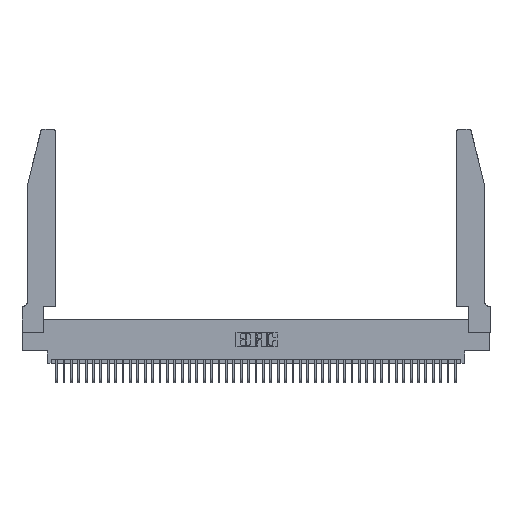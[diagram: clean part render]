
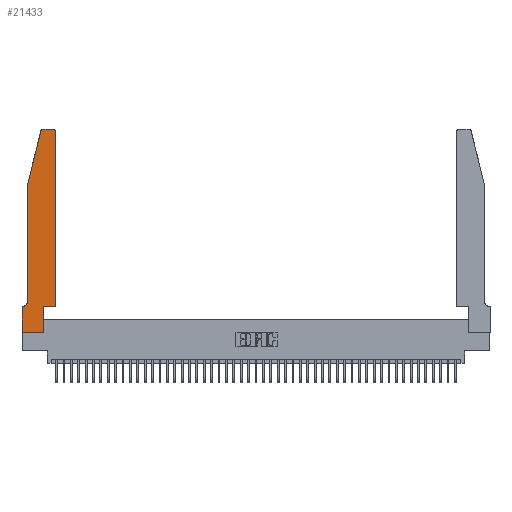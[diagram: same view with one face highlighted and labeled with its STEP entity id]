
A CAD part, top view. The second image highlights one B-rep face of the part: STEP entity #21433.
In plain terms, the highlighted planar face has unit normal (0, 0, 1).
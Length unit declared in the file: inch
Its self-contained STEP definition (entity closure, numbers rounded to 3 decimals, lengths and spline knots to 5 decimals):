
#472 = VERTEX_POINT ( 'NONE', #5790 ) ;
#1131 = LINE ( 'NONE', #6602, #27504 ) ;
#1356 = ORIENTED_EDGE ( 'NONE', *, *, #39650, .T. ) ;
#1361 = LINE ( 'NONE', #17908, #18649 ) ;
#1547 = AXIS2_PLACEMENT_3D ( 'NONE', #21243, #24685, #4097 ) ;
#2337 = CARTESIAN_POINT ( 'NONE',  ( 0.4505, 2.72, 0.37 ) ) ;
#3303 = EDGE_CURVE ( 'NONE', #12728, #18638, #10101, .T. ) ;
#3900 = AXIS2_PLACEMENT_3D ( 'NONE', #28293, #7752, #31749 ) ;
#3964 = CARTESIAN_POINT ( 'NONE',  ( 0.2865, 0.35, 0.37 ) ) ;
#4097 = DIRECTION ( 'NONE',  ( 1., 0., 0. ) ) ;
#4770 = EDGE_CURVE ( 'NONE', #28008, #28094, #12646, .T. ) ;
#5119 = DIRECTION ( 'NONE',  ( 0., 0., -1. ) ) ;
#5790 = CARTESIAN_POINT ( 'NONE',  ( 0.284, 2.75, 0.37 ) ) ;
#5871 = EDGE_CURVE ( 'NONE', #28208, #33618, #13078, .T. ) ;
#5887 = VECTOR ( 'NONE', #6612, 39.37008 ) ;
#6173 = EDGE_CURVE ( 'NONE', #33618, #11748, #1131, .T. ) ;
#6337 = ORIENTED_EDGE ( 'NONE', *, *, #6173, .T. ) ;
#6602 = CARTESIAN_POINT ( 'NONE',  ( 0.0755, 0.35, 0.37 ) ) ;
#6612 = DIRECTION ( 'NONE',  ( 1., 0., 0. ) ) ;
#7547 = CIRCLE ( 'NONE', #3900, 0.03 ) ;
#7752 = DIRECTION ( 'NONE',  ( 0., 0., 1. ) ) ;
#7864 = CARTESIAN_POINT ( 'NONE',  ( 0., 0., 0.37 ) ) ;
#7903 = AXIS2_PLACEMENT_3D ( 'NONE', #25691, #5119, #29136 ) ;
#7947 = DIRECTION ( 'NONE',  ( 0., -1., 0. ) ) ;
#8462 = CARTESIAN_POINT ( 'NONE',  ( 0., 0.35, 0.37 ) ) ;
#8558 = VECTOR ( 'NONE', #38478, 39.37008 ) ;
#9692 = EDGE_CURVE ( 'NONE', #472, #18878, #30991, .T. ) ;
#10101 = LINE ( 'NONE', #3964, #37507 ) ;
#10111 = DIRECTION ( 'NONE',  ( -1., 0., 0. ) ) ;
#10817 = DIRECTION ( 'NONE',  ( 0., 1., 0. ) ) ;
#10990 = ORIENTED_EDGE ( 'NONE', *, *, #24541, .T. ) ;
#11550 = VECTOR ( 'NONE', #34556, 39.37008 ) ;
#11748 = VERTEX_POINT ( 'NONE', #8462 ) ;
#12056 = ORIENTED_EDGE ( 'NONE', *, *, #3303, .T. ) ;
#12387 = CARTESIAN_POINT ( 'NONE',  ( 0.4505, 0.35, 0.37 ) ) ;
#12646 = LINE ( 'NONE', #26511, #21761 ) ;
#12728 = VERTEX_POINT ( 'NONE', #17555 ) ;
#13078 = CIRCLE ( 'NONE', #7903, 0.07 ) ;
#14169 = DIRECTION ( 'NONE',  ( 0., 0., 1. ) ) ;
#15694 = CARTESIAN_POINT ( 'NONE',  ( 0.0755, 2., 0.37 ) ) ;
#16012 = ORIENTED_EDGE ( 'NONE', *, *, #21445, .T. ) ;
#17079 = ORIENTED_EDGE ( 'NONE', *, *, #30278, .T. ) ;
#17509 = AXIS2_PLACEMENT_3D ( 'NONE', #34742, #14169, #38207 ) ;
#17555 = CARTESIAN_POINT ( 'NONE',  ( 0.2865, 0., 0.37 ) ) ;
#17742 = EDGE_CURVE ( 'NONE', #31681, #12728, #1361, .T. ) ;
#17771 = VERTEX_POINT ( 'NONE', #18050 ) ;
#17908 = CARTESIAN_POINT ( 'NONE',  ( 0., 0., 0.37 ) ) ;
#18050 = CARTESIAN_POINT ( 'NONE',  ( 0.4205, 2.75, 0.37 ) ) ;
#18638 = VERTEX_POINT ( 'NONE', #39473 ) ;
#18649 = VECTOR ( 'NONE', #21339, 39.37008 ) ;
#18739 = VECTOR ( 'NONE', #20151, 39.37008 ) ;
#18878 = VERTEX_POINT ( 'NONE', #34485 ) ;
#19180 = VECTOR ( 'NONE', #7947, 39.37008 ) ;
#19491 = ORIENTED_EDGE ( 'NONE', *, *, #17742, .T. ) ;
#19637 = DIRECTION ( 'NONE',  ( 0., 1., 0. ) ) ;
#20151 = DIRECTION ( 'NONE',  ( -1., 0., 0. ) ) ;
#21243 = CARTESIAN_POINT ( 'NONE',  ( 0., 0.35, 0.37 ) ) ;
#21339 = DIRECTION ( 'NONE',  ( 1., 0., 0. ) ) ;
#21433 = ADVANCED_FACE ( 'NONE', ( #44072 ), #41855, .T. ) ;
#21445 = EDGE_CURVE ( 'NONE', #28094, #17771, #7547, .T. ) ;
#21761 = VECTOR ( 'NONE', #19637, 39.37008 ) ;
#23734 = CARTESIAN_POINT ( 'NONE',  ( 0.4505, 0.35, 0.37 ) ) ;
#24541 = EDGE_CURVE ( 'NONE', #34837, #28208, #36411, .T. ) ;
#24685 = DIRECTION ( 'NONE',  ( 0., 0., 1. ) ) ;
#25691 = CARTESIAN_POINT ( 'NONE',  ( 0.0055, 0.42, 0.37 ) ) ;
#26511 = CARTESIAN_POINT ( 'NONE',  ( 0.4505, 0.35, 0.37 ) ) ;
#27504 = VECTOR ( 'NONE', #10111, 39.37008 ) ;
#28008 = VERTEX_POINT ( 'NONE', #12387 ) ;
#28094 = VERTEX_POINT ( 'NONE', #2337 ) ;
#28208 = VERTEX_POINT ( 'NONE', #44320 ) ;
#28293 = CARTESIAN_POINT ( 'NONE',  ( 0.4205, 2.72, 0.37 ) ) ;
#28480 = CARTESIAN_POINT ( 'NONE',  ( 0.0755, 2., 0.37 ) ) ;
#29136 = DIRECTION ( 'NONE',  ( -1., 0., 0. ) ) ;
#29721 = LINE ( 'NONE', #31052, #11550 ) ;
#30278 = EDGE_CURVE ( 'NONE', #18878, #34837, #29721, .T. ) ;
#30991 = CIRCLE ( 'NONE', #17509, 0.03 ) ;
#31052 = CARTESIAN_POINT ( 'NONE',  ( 0.0755, 2., 0.37 ) ) ;
#31518 = CARTESIAN_POINT ( 'NONE',  ( 0., 0., 0.37 ) ) ;
#31681 = VERTEX_POINT ( 'NONE', #7864 ) ;
#31749 = DIRECTION ( 'NONE',  ( 1., 0., 0. ) ) ;
#32219 = ORIENTED_EDGE ( 'NONE', *, *, #4770, .T. ) ;
#33319 = LINE ( 'NONE', #23734, #5887 ) ;
#33618 = VERTEX_POINT ( 'NONE', #33641 ) ;
#33641 = CARTESIAN_POINT ( 'NONE',  ( 0.0055, 0.35, 0.37 ) ) ;
#33838 = CARTESIAN_POINT ( 'NONE',  ( 0.2605, 2.75, 0.37 ) ) ;
#34485 = CARTESIAN_POINT ( 'NONE',  ( 0.25487, 2.72718, 0.37 ) ) ;
#34556 = DIRECTION ( 'NONE',  ( -0.239, -0.971, 0. ) ) ;
#34742 = CARTESIAN_POINT ( 'NONE',  ( 0.284, 2.72, 0.37 ) ) ;
#34837 = VERTEX_POINT ( 'NONE', #15694 ) ;
#36327 = ORIENTED_EDGE ( 'NONE', *, *, #9692, .T. ) ;
#36411 = LINE ( 'NONE', #28480, #19180 ) ;
#36845 = ORIENTED_EDGE ( 'NONE', *, *, #43450, .T. ) ;
#37042 = LINE ( 'NONE', #31518, #8558 ) ;
#37507 = VECTOR ( 'NONE', #10817, 39.37008 ) ;
#38107 = LINE ( 'NONE', #33838, #18739 ) ;
#38207 = DIRECTION ( 'NONE',  ( 1., 0., 0. ) ) ;
#38478 = DIRECTION ( 'NONE',  ( 0., -1., 0. ) ) ;
#38681 = EDGE_CURVE ( 'NONE', #18638, #28008, #33319, .T. ) ;
#38729 = EDGE_LOOP ( 'NONE', ( #1356, #36327, #17079, #10990, #41504, #6337, #36845, #19491, #12056, #44178, #32219, #16012 ) ) ;
#39473 = CARTESIAN_POINT ( 'NONE',  ( 0.2865, 0.35, 0.37 ) ) ;
#39650 = EDGE_CURVE ( 'NONE', #17771, #472, #38107, .T. ) ;
#41504 = ORIENTED_EDGE ( 'NONE', *, *, #5871, .T. ) ;
#41855 = PLANE ( 'NONE',  #1547 ) ;
#43450 = EDGE_CURVE ( 'NONE', #11748, #31681, #37042, .T. ) ;
#44072 = FACE_OUTER_BOUND ( 'NONE', #38729, .T. ) ;
#44178 = ORIENTED_EDGE ( 'NONE', *, *, #38681, .T. ) ;
#44320 = CARTESIAN_POINT ( 'NONE',  ( 0.0755, 0.42, 0.37 ) ) ;
